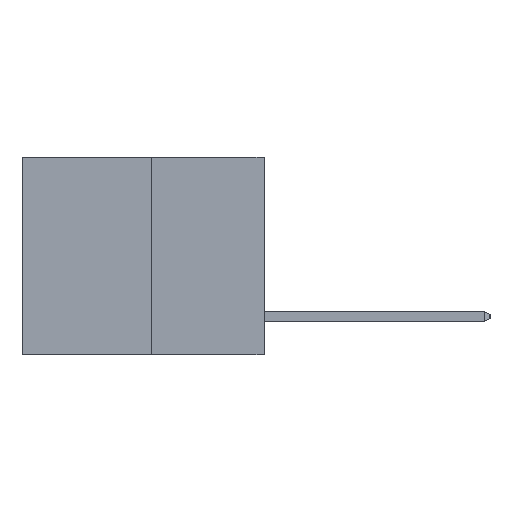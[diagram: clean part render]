
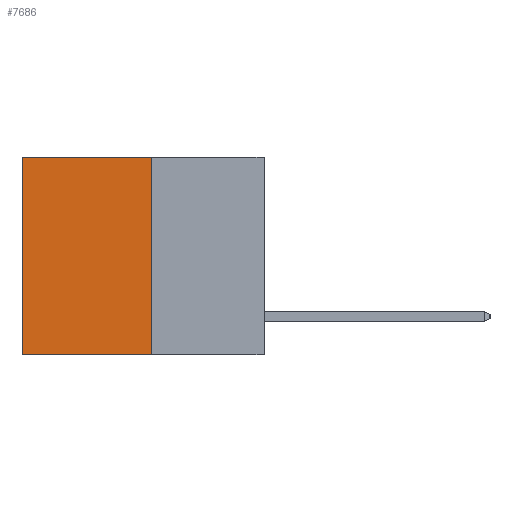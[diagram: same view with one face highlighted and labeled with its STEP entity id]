
A CAD part, left-side view. The second image highlights one B-rep face of the part: STEP entity #7686.
In plain terms, the highlighted planar face has unit normal (-1, 0, 0).
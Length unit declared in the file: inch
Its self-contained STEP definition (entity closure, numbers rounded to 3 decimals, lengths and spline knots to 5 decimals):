
#113 = DIRECTION ( 'NONE',  ( 1., 0., 0. ) ) ;
#264 = EDGE_CURVE ( 'NONE', #10621, #10236, #13160, .T. ) ;
#294 = ORIENTED_EDGE ( 'NONE', *, *, #264, .T. ) ;
#298 = DIRECTION ( 'NONE',  ( 0., 0., -1. ) ) ;
#725 = LINE ( 'NONE', #11771, #3095 ) ;
#1676 = VECTOR ( 'NONE', #11001, 39.37008 ) ;
#1743 = CARTESIAN_POINT ( 'NONE',  ( 0.3165, 0.28, -0.49 ) ) ;
#1832 = VERTEX_POINT ( 'NONE', #6710 ) ;
#1871 = ORIENTED_EDGE ( 'NONE', *, *, #3619, .T. ) ;
#2175 = CARTESIAN_POINT ( 'NONE',  ( 0.3165, 0.6, -0.49 ) ) ;
#2497 = ORIENTED_EDGE ( 'NONE', *, *, #8461, .F. ) ;
#2917 = ORIENTED_EDGE ( 'NONE', *, *, #4963, .F. ) ;
#3095 = VECTOR ( 'NONE', #6510, 39.37008 ) ;
#3297 = VECTOR ( 'NONE', #10867, 39.37008 ) ;
#3619 = EDGE_CURVE ( 'NONE', #13027, #10621, #10161, .T. ) ;
#4963 = EDGE_CURVE ( 'NONE', #13027, #1832, #725, .T. ) ;
#5177 = LINE ( 'NONE', #1743, #3297 ) ;
#6269 = CARTESIAN_POINT ( 'NONE',  ( 0.3165, 0.28, -0.49 ) ) ;
#6480 = CARTESIAN_POINT ( 'NONE',  ( 0.3165, 0.6, -0.49 ) ) ;
#6510 = DIRECTION ( 'NONE',  ( 0., 0., -1. ) ) ;
#6710 = CARTESIAN_POINT ( 'NONE',  ( 0.3165, 0.28, -0.49 ) ) ;
#6847 = CARTESIAN_POINT ( 'NONE',  ( 0.3165, 0.6, 0. ) ) ;
#6868 = CARTESIAN_POINT ( 'NONE',  ( 0.3165, 0.28, 0. ) ) ;
#6995 = VECTOR ( 'NONE', #12790, 39.37008 ) ;
#7686 = ADVANCED_FACE ( 'NONE', ( #12242 ), #8376, .F. ) ;
#8376 = PLANE ( 'NONE',  #9483 ) ;
#8461 = EDGE_CURVE ( 'NONE', #1832, #10236, #5177, .T. ) ;
#9483 = AXIS2_PLACEMENT_3D ( 'NONE', #6269, #113, #298 ) ;
#10161 = LINE ( 'NONE', #10654, #6995 ) ;
#10236 = VERTEX_POINT ( 'NONE', #6480 ) ;
#10621 = VERTEX_POINT ( 'NONE', #6847 ) ;
#10654 = CARTESIAN_POINT ( 'NONE',  ( 0.3165, 0.28, 0. ) ) ;
#10867 = DIRECTION ( 'NONE',  ( 0., 1., 0. ) ) ;
#11001 = DIRECTION ( 'NONE',  ( 0., 0., -1. ) ) ;
#11078 = EDGE_LOOP ( 'NONE', ( #294, #2497, #2917, #1871 ) ) ;
#11771 = CARTESIAN_POINT ( 'NONE',  ( 0.3165, 0.28, -0.49 ) ) ;
#12242 = FACE_OUTER_BOUND ( 'NONE', #11078, .T. ) ;
#12790 = DIRECTION ( 'NONE',  ( 0., 1., 0. ) ) ;
#13027 = VERTEX_POINT ( 'NONE', #6868 ) ;
#13160 = LINE ( 'NONE', #2175, #1676 ) ;
